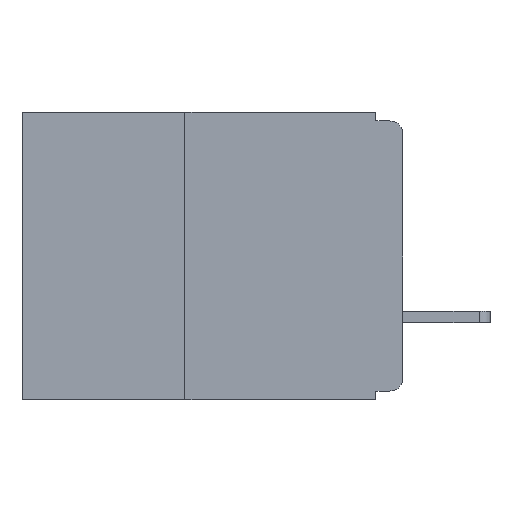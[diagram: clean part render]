
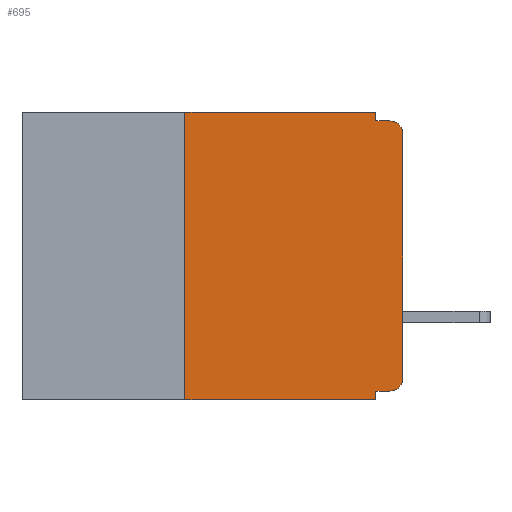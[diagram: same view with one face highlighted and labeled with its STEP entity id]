
A CAD part, left-side view. The second image highlights one B-rep face of the part: STEP entity #695.
In plain terms, the highlighted planar face has unit normal (-1, 0, 0).
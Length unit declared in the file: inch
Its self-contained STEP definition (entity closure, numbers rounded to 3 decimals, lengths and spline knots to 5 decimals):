
#225 = CARTESIAN_POINT ( 'NONE',  ( 0., 0.031, 0. ) ) ;
#300 = AXIS2_PLACEMENT_3D ( 'NONE', #4840, #3050, #10127 ) ;
#689 = EDGE_CURVE ( 'NONE', #9916, #10174, #2119, .T. ) ;
#695 = ADVANCED_FACE ( 'NONE', ( #2002 ), #800, .F. ) ;
#768 = CARTESIAN_POINT ( 'NONE',  ( 0., 0.031, -0.33 ) ) ;
#800 = PLANE ( 'NONE',  #300 ) ;
#1597 = VERTEX_POINT ( 'NONE', #10658 ) ;
#1736 = VERTEX_POINT ( 'NONE', #9542 ) ;
#1895 = CARTESIAN_POINT ( 'NONE',  ( 0., 0.015, -0.01 ) ) ;
#2002 = FACE_OUTER_BOUND ( 'NONE', #8400, .T. ) ;
#2030 = VECTOR ( 'NONE', #6943, 39.37008 ) ;
#2119 = LINE ( 'NONE', #10175, #2030 ) ;
#2625 = DIRECTION ( 'NONE',  ( 0., 0., -1. ) ) ;
#2634 = DIRECTION ( 'NONE',  ( -1., 0., 0. ) ) ;
#2651 = CARTESIAN_POINT ( 'NONE',  ( 0., 0.015, -0.305 ) ) ;
#2984 = DIRECTION ( 'NONE',  ( 0., 0., -1. ) ) ;
#3013 = DIRECTION ( 'NONE',  ( -1., 0., 0. ) ) ;
#3014 = CARTESIAN_POINT ( 'NONE',  ( 0., 0.015, -0.025 ) ) ;
#3050 = DIRECTION ( 'NONE',  ( 1., 0., 0. ) ) ;
#3362 = DIRECTION ( 'NONE',  ( 0., 1., 0. ) ) ;
#3395 = CARTESIAN_POINT ( 'NONE',  ( 0., 0., -0.32 ) ) ;
#3455 = CARTESIAN_POINT ( 'NONE',  ( 0., 0.031, -0.01 ) ) ;
#3640 = CARTESIAN_POINT ( 'NONE',  ( 0., 0.015, -0.32 ) ) ;
#3718 = DIRECTION ( 'NONE',  ( 0., -1., 0. ) ) ;
#3734 = CARTESIAN_POINT ( 'NONE',  ( 0., 0., -0.025 ) ) ;
#3735 = CARTESIAN_POINT ( 'NONE',  ( 0., 0., -0.01 ) ) ;
#4415 = CARTESIAN_POINT ( 'NONE',  ( 0., 0., -0.305 ) ) ;
#4435 = VECTOR ( 'NONE', #10675, 39.37008 ) ;
#4472 = VECTOR ( 'NONE', #10813, 39.37008 ) ;
#4586 = CARTESIAN_POINT ( 'NONE',  ( 0., 0., 0. ) ) ;
#4588 = LINE ( 'NONE', #10694, #4435 ) ;
#4595 = VECTOR ( 'NONE', #10907, 39.37008 ) ;
#4632 = LINE ( 'NONE', #10937, #4595 ) ;
#4639 = DIRECTION ( 'NONE',  ( 0., 0., 1. ) ) ;
#4681 = VECTOR ( 'NONE', #10846, 39.37008 ) ;
#4780 = LINE ( 'NONE', #10912, #4472 ) ;
#4840 = CARTESIAN_POINT ( 'NONE',  ( 0., 0.437, 0. ) ) ;
#5112 = LINE ( 'NONE', #10968, #4681 ) ;
#5811 = AXIS2_PLACEMENT_3D ( 'NONE', #2651, #2634, #2625 ) ;
#5865 = CARTESIAN_POINT ( 'NONE',  ( 0., 0.25, 0. ) ) ;
#5923 = EDGE_CURVE ( 'NONE', #9989, #8941, #9922, .T. ) ;
#5987 = EDGE_CURVE ( 'NONE', #8167, #6571, #9532, .T. ) ;
#6034 = EDGE_CURVE ( 'NONE', #8953, #1597, #9329, .T. ) ;
#6087 = EDGE_CURVE ( 'NONE', #8941, #6571, #9234, .T. ) ;
#6106 = EDGE_CURVE ( 'NONE', #8953, #9989, #9097, .T. ) ;
#6571 = VERTEX_POINT ( 'NONE', #1895 ) ;
#6699 = EDGE_CURVE ( 'NONE', #10174, #8167, #4632, .T. ) ;
#6700 = EDGE_CURVE ( 'NONE', #1736, #9916, #5112, .T. ) ;
#6736 = EDGE_CURVE ( 'NONE', #1736, #9167, #4780, .T. ) ;
#6753 = EDGE_CURVE ( 'NONE', #1597, #9167, #4588, .T. ) ;
#6943 = DIRECTION ( 'NONE',  ( 0., -1., 0. ) ) ;
#8167 = VERTEX_POINT ( 'NONE', #3455 ) ;
#8400 = EDGE_LOOP ( 'NONE', ( #8973, #9030, #9139, #9242, #10421, #10449, #10488, #10667, #10696, #10736 ) ) ;
#8873 = AXIS2_PLACEMENT_3D ( 'NONE', #3014, #3013, #2984 ) ;
#8941 = VERTEX_POINT ( 'NONE', #3734 ) ;
#8953 = VERTEX_POINT ( 'NONE', #3640 ) ;
#8973 = ORIENTED_EDGE ( 'NONE', *, *, #5923, .T. ) ;
#9030 = ORIENTED_EDGE ( 'NONE', *, *, #6087, .T. ) ;
#9097 = CIRCLE ( 'NONE', #5811, 0.015 ) ;
#9139 = ORIENTED_EDGE ( 'NONE', *, *, #5987, .F. ) ;
#9167 = VERTEX_POINT ( 'NONE', #768 ) ;
#9234 = CIRCLE ( 'NONE', #8873, 0.015 ) ;
#9242 = ORIENTED_EDGE ( 'NONE', *, *, #6699, .F. ) ;
#9329 = LINE ( 'NONE', #3395, #9431 ) ;
#9431 = VECTOR ( 'NONE', #3362, 39.37008 ) ;
#9532 = LINE ( 'NONE', #3735, #9584 ) ;
#9542 = CARTESIAN_POINT ( 'NONE',  ( 0., 0.25, -0.33 ) ) ;
#9584 = VECTOR ( 'NONE', #3718, 39.37008 ) ;
#9714 = VECTOR ( 'NONE', #4639, 39.37008 ) ;
#9916 = VERTEX_POINT ( 'NONE', #5865 ) ;
#9922 = LINE ( 'NONE', #4586, #9714 ) ;
#9989 = VERTEX_POINT ( 'NONE', #4415 ) ;
#10127 = DIRECTION ( 'NONE',  ( 0., 0., -1. ) ) ;
#10174 = VERTEX_POINT ( 'NONE', #225 ) ;
#10175 = CARTESIAN_POINT ( 'NONE',  ( 0., 0.437, 0. ) ) ;
#10421 = ORIENTED_EDGE ( 'NONE', *, *, #689, .F. ) ;
#10449 = ORIENTED_EDGE ( 'NONE', *, *, #6700, .F. ) ;
#10488 = ORIENTED_EDGE ( 'NONE', *, *, #6736, .T. ) ;
#10658 = CARTESIAN_POINT ( 'NONE',  ( 0., 0.031, -0.32 ) ) ;
#10667 = ORIENTED_EDGE ( 'NONE', *, *, #6753, .F. ) ;
#10675 = DIRECTION ( 'NONE',  ( 0., 0., -1. ) ) ;
#10694 = CARTESIAN_POINT ( 'NONE',  ( 0., 0.031, -0.33 ) ) ;
#10696 = ORIENTED_EDGE ( 'NONE', *, *, #6034, .F. ) ;
#10736 = ORIENTED_EDGE ( 'NONE', *, *, #6106, .T. ) ;
#10813 = DIRECTION ( 'NONE',  ( 0., -1., 0. ) ) ;
#10846 = DIRECTION ( 'NONE',  ( 0., 0., 1. ) ) ;
#10907 = DIRECTION ( 'NONE',  ( 0., 0., -1. ) ) ;
#10912 = CARTESIAN_POINT ( 'NONE',  ( 0., 0.437, -0.33 ) ) ;
#10937 = CARTESIAN_POINT ( 'NONE',  ( 0., 0.031, 0. ) ) ;
#10968 = CARTESIAN_POINT ( 'NONE',  ( 0., 0.25, -0.33 ) ) ;
